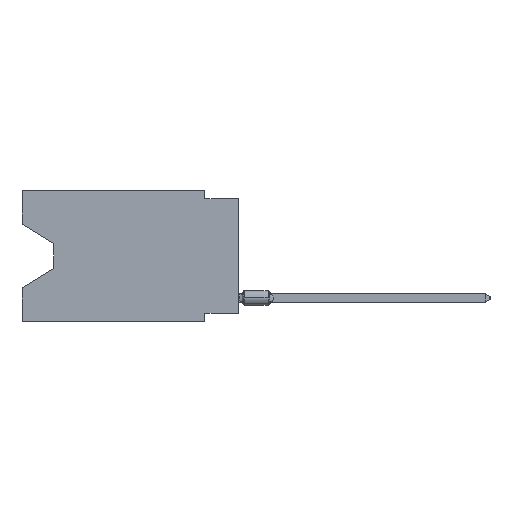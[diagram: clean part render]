
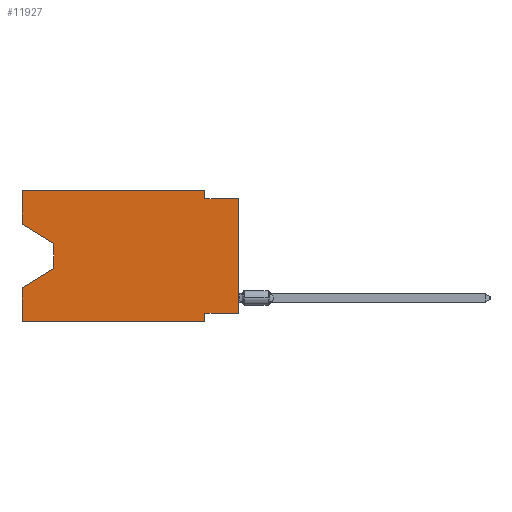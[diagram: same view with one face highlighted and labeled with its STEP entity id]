
A CAD part, left-side view. The second image highlights one B-rep face of the part: STEP entity #11927.
In plain terms, the highlighted planar face has unit normal (-1, 0, 0).
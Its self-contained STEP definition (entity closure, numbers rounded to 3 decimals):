
#1072 = DIRECTION ( 'NONE',  ( 0., 0., 1. ) ) ;
#1454 = ORIENTED_EDGE ( 'NONE', *, *, #28989, .T. ) ;
#1651 = VERTEX_POINT ( 'NONE', #3145 ) ;
#1765 = VERTEX_POINT ( 'NONE', #34941 ) ;
#1774 = LINE ( 'NONE', #9524, #6703 ) ;
#2413 = VERTEX_POINT ( 'NONE', #21793 ) ;
#2889 = LINE ( 'NONE', #23454, #12665 ) ;
#3098 = DIRECTION ( 'NONE',  ( 0., -1., 0. ) ) ;
#3145 = CARTESIAN_POINT ( 'NONE',  ( 0., 16.383, 0. ) ) ;
#3304 = VECTOR ( 'NONE', #25953, 1000. ) ;
#3801 = ORIENTED_EDGE ( 'NONE', *, *, #32008, .F. ) ;
#4389 = VERTEX_POINT ( 'NONE', #37198 ) ;
#6173 = EDGE_CURVE ( 'NONE', #1651, #22928, #2889, .T. ) ;
#6254 = CARTESIAN_POINT ( 'NONE',  ( 0., 0., -9.271 ) ) ;
#6348 = DIRECTION ( 'NONE',  ( 0., 0., -1. ) ) ;
#6520 = CARTESIAN_POINT ( 'NONE',  ( 0., 0., -0.635 ) ) ;
#6703 = VECTOR ( 'NONE', #40261, 1000. ) ;
#6787 = PLANE ( 'NONE',  #41223 ) ;
#8150 = VERTEX_POINT ( 'NONE', #17333 ) ;
#8793 = LINE ( 'NONE', #6254, #33450 ) ;
#9212 = CARTESIAN_POINT ( 'NONE',  ( 0., 16.383, -9.906 ) ) ;
#9524 = CARTESIAN_POINT ( 'NONE',  ( 0., 2.54, -9.906 ) ) ;
#10899 = DIRECTION ( 'NONE',  ( 0., 0., -1. ) ) ;
#10901 = CARTESIAN_POINT ( 'NONE',  ( 0., 13.97, -4.013 ) ) ;
#11101 = ORIENTED_EDGE ( 'NONE', *, *, #32838, .F. ) ;
#11284 = CARTESIAN_POINT ( 'NONE',  ( 0., 16.383, 0. ) ) ;
#11927 = ADVANCED_FACE ( 'NONE', ( #23349 ), #6787, .F. ) ;
#12293 = EDGE_CURVE ( 'NONE', #12920, #2413, #43518, .T. ) ;
#12665 = VECTOR ( 'NONE', #3098, 1000. ) ;
#12852 = VERTEX_POINT ( 'NONE', #14655 ) ;
#12920 = VERTEX_POINT ( 'NONE', #26058 ) ;
#13854 = VERTEX_POINT ( 'NONE', #19890 ) ;
#13877 = DIRECTION ( 'NONE',  ( 0., -1., 0. ) ) ;
#14490 = LINE ( 'NONE', #18076, #25883 ) ;
#14655 = CARTESIAN_POINT ( 'NONE',  ( 0., 2.54, -9.271 ) ) ;
#15048 = ORIENTED_EDGE ( 'NONE', *, *, #37317, .F. ) ;
#16192 = CARTESIAN_POINT ( 'NONE',  ( 0., 16.383, 0. ) ) ;
#16308 = VECTOR ( 'NONE', #13877, 1000. ) ;
#16360 = VECTOR ( 'NONE', #21533, 1000. ) ;
#17333 = CARTESIAN_POINT ( 'NONE',  ( 0., 16.383, -7.36 ) ) ;
#17615 = LINE ( 'NONE', #37810, #34798 ) ;
#18062 = LINE ( 'NONE', #10901, #30919 ) ;
#18076 = CARTESIAN_POINT ( 'NONE',  ( 0., 16.383, 0. ) ) ;
#19890 = CARTESIAN_POINT ( 'NONE',  ( 0., 0., -0.635 ) ) ;
#20452 = VECTOR ( 'NONE', #32953, 1000. ) ;
#21313 = ORIENTED_EDGE ( 'NONE', *, *, #34672, .F. ) ;
#21533 = DIRECTION ( 'NONE',  ( 0., 0.855, -0.519 ) ) ;
#21793 = CARTESIAN_POINT ( 'NONE',  ( 0., 2.54, -9.906 ) ) ;
#22228 = ORIENTED_EDGE ( 'NONE', *, *, #12293, .T. ) ;
#22928 = VERTEX_POINT ( 'NONE', #27957 ) ;
#23349 = FACE_OUTER_BOUND ( 'NONE', #27915, .T. ) ;
#23454 = CARTESIAN_POINT ( 'NONE',  ( 0., 16.383, 0. ) ) ;
#24663 = EDGE_CURVE ( 'NONE', #4389, #1651, #14490, .T. ) ;
#24772 = ORIENTED_EDGE ( 'NONE', *, *, #27312, .T. ) ;
#25291 = ORIENTED_EDGE ( 'NONE', *, *, #24663, .F. ) ;
#25387 = LINE ( 'NONE', #11284, #41727 ) ;
#25883 = VECTOR ( 'NONE', #1072, 1000. ) ;
#25953 = DIRECTION ( 'NONE',  ( 0., -0.855, -0.519 ) ) ;
#26058 = CARTESIAN_POINT ( 'NONE',  ( 0., 16.383, -9.906 ) ) ;
#26092 = VERTEX_POINT ( 'NONE', #35562 ) ;
#26758 = CARTESIAN_POINT ( 'NONE',  ( 0., 13.97, -5.893 ) ) ;
#27312 = EDGE_CURVE ( 'NONE', #39519, #8150, #39255, .T. ) ;
#27915 = EDGE_LOOP ( 'NONE', ( #1454, #42787, #24772, #3801, #22228, #11101, #15048, #41714, #31136, #21313, #35995, #25291 ) ) ;
#27957 = CARTESIAN_POINT ( 'NONE',  ( 0., 2.54, 0. ) ) ;
#28989 = EDGE_CURVE ( 'NONE', #4389, #44028, #36273, .T. ) ;
#29380 = EDGE_CURVE ( 'NONE', #1765, #13854, #17615, .T. ) ;
#29585 = VECTOR ( 'NONE', #10899, 1000. ) ;
#29861 = DIRECTION ( 'NONE',  ( 1., 0., 0. ) ) ;
#29985 = CARTESIAN_POINT ( 'NONE',  ( 0., 16.383, -2.546 ) ) ;
#30697 = LINE ( 'NONE', #6520, #16308 ) ;
#30919 = VECTOR ( 'NONE', #34879, 1000. ) ;
#31064 = DIRECTION ( 'NONE',  ( 0., 0., 1. ) ) ;
#31136 = ORIENTED_EDGE ( 'NONE', *, *, #42541, .F. ) ;
#31373 = EDGE_CURVE ( 'NONE', #44028, #39519, #18062, .T. ) ;
#32008 = EDGE_CURVE ( 'NONE', #12920, #8150, #25387, .T. ) ;
#32838 = EDGE_CURVE ( 'NONE', #12852, #2413, #1774, .T. ) ;
#32953 = DIRECTION ( 'NONE',  ( 0., -1., 0. ) ) ;
#33450 = VECTOR ( 'NONE', #33814, 1000. ) ;
#33799 = CARTESIAN_POINT ( 'NONE',  ( 0., 13.97, -4.013 ) ) ;
#33814 = DIRECTION ( 'NONE',  ( 0., 1., 0. ) ) ;
#34672 = EDGE_CURVE ( 'NONE', #22928, #26092, #42079, .T. ) ;
#34798 = VECTOR ( 'NONE', #31064, 1000. ) ;
#34879 = DIRECTION ( 'NONE',  ( 0., 0., -1. ) ) ;
#34941 = CARTESIAN_POINT ( 'NONE',  ( 0., 0., -9.271 ) ) ;
#35112 = CARTESIAN_POINT ( 'NONE',  ( 0., 2.54, 0. ) ) ;
#35562 = CARTESIAN_POINT ( 'NONE',  ( 0., 2.54, -0.635 ) ) ;
#35995 = ORIENTED_EDGE ( 'NONE', *, *, #6173, .F. ) ;
#36273 = LINE ( 'NONE', #29985, #3304 ) ;
#37198 = CARTESIAN_POINT ( 'NONE',  ( 0., 16.383, -2.546 ) ) ;
#37317 = EDGE_CURVE ( 'NONE', #1765, #12852, #8793, .T. ) ;
#37810 = CARTESIAN_POINT ( 'NONE',  ( 0., 0., 0. ) ) ;
#39028 = CARTESIAN_POINT ( 'NONE',  ( 0., 13.97, -5.893 ) ) ;
#39093 = DIRECTION ( 'NONE',  ( 0., 0., 1. ) ) ;
#39255 = LINE ( 'NONE', #39028, #16360 ) ;
#39519 = VERTEX_POINT ( 'NONE', #26758 ) ;
#40261 = DIRECTION ( 'NONE',  ( 0., 0., -1. ) ) ;
#41223 = AXIS2_PLACEMENT_3D ( 'NONE', #16192, #29861, #6348 ) ;
#41714 = ORIENTED_EDGE ( 'NONE', *, *, #29380, .T. ) ;
#41727 = VECTOR ( 'NONE', #39093, 1000. ) ;
#42079 = LINE ( 'NONE', #35112, #29585 ) ;
#42541 = EDGE_CURVE ( 'NONE', #26092, #13854, #30697, .T. ) ;
#42787 = ORIENTED_EDGE ( 'NONE', *, *, #31373, .T. ) ;
#43518 = LINE ( 'NONE', #9212, #20452 ) ;
#44028 = VERTEX_POINT ( 'NONE', #33799 ) ;
